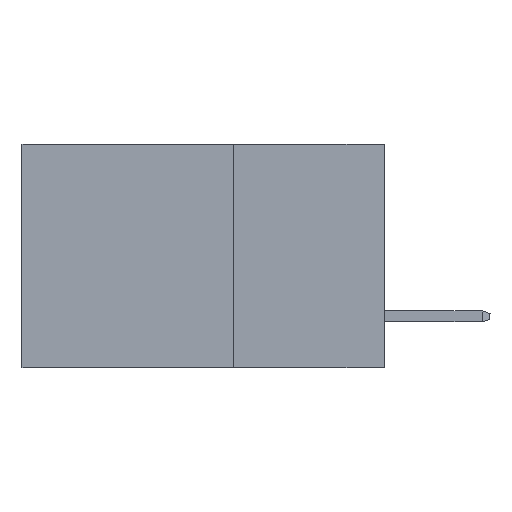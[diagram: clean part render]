
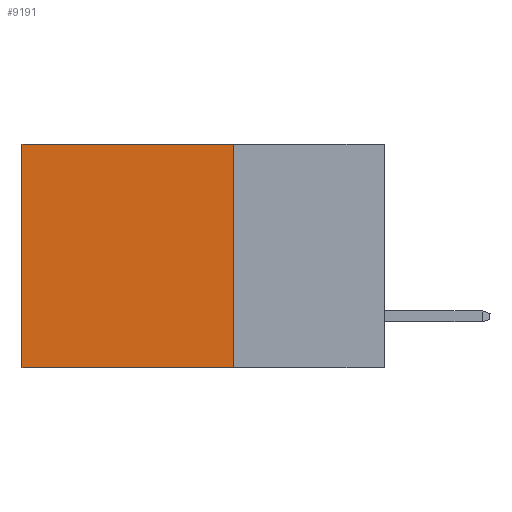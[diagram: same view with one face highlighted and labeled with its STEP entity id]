
A CAD part, left-side view. The second image highlights one B-rep face of the part: STEP entity #9191.
In plain terms, the highlighted planar face has unit normal (-1, 0, 0).
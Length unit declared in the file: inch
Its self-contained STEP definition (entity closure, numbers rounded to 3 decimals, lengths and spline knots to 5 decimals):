
#139 = VERTEX_POINT ( 'NONE', #4547 ) ;
#758 = CARTESIAN_POINT ( 'NONE',  ( 0.2615, 0.6, -0.37 ) ) ;
#828 = EDGE_CURVE ( 'NONE', #6080, #9426, #13489, .T. ) ;
#838 = EDGE_CURVE ( 'NONE', #9426, #139, #14391, .T. ) ;
#1291 = ORIENTED_EDGE ( 'NONE', *, *, #838, .T. ) ;
#1767 = ORIENTED_EDGE ( 'NONE', *, *, #828, .T. ) ;
#2273 = CARTESIAN_POINT ( 'NONE',  ( 0.2615, 0.25, -0.37 ) ) ;
#2387 = AXIS2_PLACEMENT_3D ( 'NONE', #2273, #11527, #8040 ) ;
#2554 = LINE ( 'NONE', #3653, #7941 ) ;
#3653 = CARTESIAN_POINT ( 'NONE',  ( 0.2615, 0.25, -0.37 ) ) ;
#4320 = CARTESIAN_POINT ( 'NONE',  ( 0.2615, 0.25, 0. ) ) ;
#4547 = CARTESIAN_POINT ( 'NONE',  ( 0.2615, 0.6, -0.37 ) ) ;
#5005 = DIRECTION ( 'NONE',  ( 0., 1., 0. ) ) ;
#5416 = VECTOR ( 'NONE', #12195, 39.37008 ) ;
#6080 = VERTEX_POINT ( 'NONE', #4320 ) ;
#6751 = VECTOR ( 'NONE', #8364, 39.37008 ) ;
#7170 = LINE ( 'NONE', #11777, #6751 ) ;
#7201 = EDGE_CURVE ( 'NONE', #8912, #139, #2554, .T. ) ;
#7941 = VECTOR ( 'NONE', #5005, 39.37008 ) ;
#8040 = DIRECTION ( 'NONE',  ( 0., 0., -1. ) ) ;
#8364 = DIRECTION ( 'NONE',  ( 0., 0., -1. ) ) ;
#8912 = VERTEX_POINT ( 'NONE', #11020 ) ;
#9191 = ADVANCED_FACE ( 'NONE', ( #11601 ), #13898, .F. ) ;
#9426 = VERTEX_POINT ( 'NONE', #11893 ) ;
#11020 = CARTESIAN_POINT ( 'NONE',  ( 0.2615, 0.25, -0.37 ) ) ;
#11201 = VECTOR ( 'NONE', #12123, 39.37008 ) ;
#11222 = CARTESIAN_POINT ( 'NONE',  ( 0.2615, 0.25, 0. ) ) ;
#11478 = ORIENTED_EDGE ( 'NONE', *, *, #13051, .F. ) ;
#11527 = DIRECTION ( 'NONE',  ( 1., 0., 0. ) ) ;
#11601 = FACE_OUTER_BOUND ( 'NONE', #14709, .T. ) ;
#11777 = CARTESIAN_POINT ( 'NONE',  ( 0.2615, 0.25, -0.37 ) ) ;
#11893 = CARTESIAN_POINT ( 'NONE',  ( 0.2615, 0.6, 0. ) ) ;
#12123 = DIRECTION ( 'NONE',  ( 0., 0., -1. ) ) ;
#12195 = DIRECTION ( 'NONE',  ( 0., 1., 0. ) ) ;
#13051 = EDGE_CURVE ( 'NONE', #6080, #8912, #7170, .T. ) ;
#13489 = LINE ( 'NONE', #11222, #5416 ) ;
#13898 = PLANE ( 'NONE',  #2387 ) ;
#14391 = LINE ( 'NONE', #758, #11201 ) ;
#14665 = ORIENTED_EDGE ( 'NONE', *, *, #7201, .F. ) ;
#14709 = EDGE_LOOP ( 'NONE', ( #1291, #14665, #11478, #1767 ) ) ;
